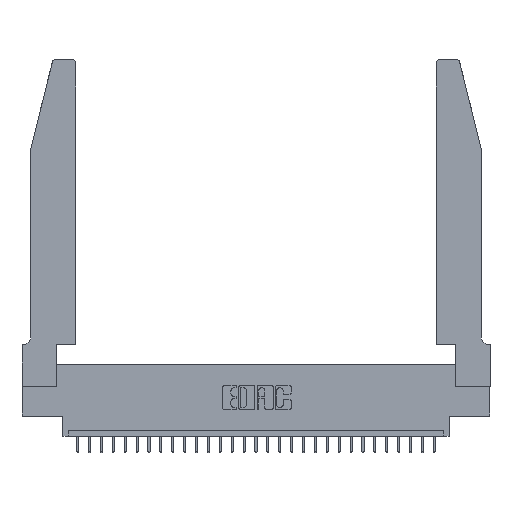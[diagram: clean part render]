
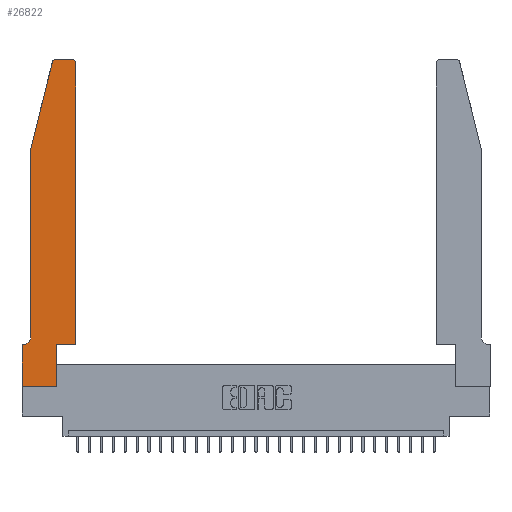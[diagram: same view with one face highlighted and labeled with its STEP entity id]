
A CAD part, top view. The second image highlights one B-rep face of the part: STEP entity #26822.
In plain terms, the highlighted planar face has unit normal (0, 0, 1).
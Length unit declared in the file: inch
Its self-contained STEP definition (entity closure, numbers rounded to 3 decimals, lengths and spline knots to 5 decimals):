
#91 = CARTESIAN_POINT ( 'NONE',  ( 0.4505, 0.35, 0.37 ) ) ;
#554 = CARTESIAN_POINT ( 'NONE',  ( 0.2865, 0.35, 0.37 ) ) ;
#603 = CARTESIAN_POINT ( 'NONE',  ( 0., 0., 0.37 ) ) ;
#962 = VECTOR ( 'NONE', #23819, 39.37008 ) ;
#1240 = VECTOR ( 'NONE', #25813, 39.37008 ) ;
#1410 = VECTOR ( 'NONE', #29481, 39.37008 ) ;
#1724 = ORIENTED_EDGE ( 'NONE', *, *, #6148, .T. ) ;
#1778 = DIRECTION ( 'NONE',  ( 0., 0., -1. ) ) ;
#2444 = PLANE ( 'NONE',  #16899 ) ;
#2586 = FACE_OUTER_BOUND ( 'NONE', #18977, .T. ) ;
#2711 = CARTESIAN_POINT ( 'NONE',  ( 0.284, 2.75, 0.37 ) ) ;
#2952 = DIRECTION ( 'NONE',  ( 1., 0., 0. ) ) ;
#3609 = CARTESIAN_POINT ( 'NONE',  ( 0.0055, 0.42, 0.37 ) ) ;
#3892 = DIRECTION ( 'NONE',  ( -1., 0., 0. ) ) ;
#3973 = VERTEX_POINT ( 'NONE', #24589 ) ;
#4111 = VERTEX_POINT ( 'NONE', #554 ) ;
#4314 = LINE ( 'NONE', #23002, #27967 ) ;
#4425 = CARTESIAN_POINT ( 'NONE',  ( 0.25487, 2.72718, 0.37 ) ) ;
#4513 = EDGE_CURVE ( 'NONE', #6541, #19945, #12818, .T. ) ;
#4769 = ORIENTED_EDGE ( 'NONE', *, *, #24061, .T. ) ;
#4992 = DIRECTION ( 'NONE',  ( 0., 0., 1. ) ) ;
#5116 = CARTESIAN_POINT ( 'NONE',  ( 0.2865, 0.35, 0.37 ) ) ;
#5364 = EDGE_CURVE ( 'NONE', #3973, #4111, #9200, .T. ) ;
#6148 = EDGE_CURVE ( 'NONE', #21252, #3973, #9681, .T. ) ;
#6361 = CARTESIAN_POINT ( 'NONE',  ( 0.284, 2.72, 0.37 ) ) ;
#6541 = VERTEX_POINT ( 'NONE', #2711 ) ;
#7515 = CARTESIAN_POINT ( 'NONE',  ( 0., 0.35, 0.37 ) ) ;
#7552 = LINE ( 'NONE', #603, #962 ) ;
#7604 = ORIENTED_EDGE ( 'NONE', *, *, #14848, .T. ) ;
#8193 = VECTOR ( 'NONE', #8995, 39.37008 ) ;
#8543 = VERTEX_POINT ( 'NONE', #29185 ) ;
#8554 = LINE ( 'NONE', #24541, #28881 ) ;
#8576 = CIRCLE ( 'NONE', #17254, 0.07 ) ;
#8995 = DIRECTION ( 'NONE',  ( 0., -1., 0. ) ) ;
#9142 = CARTESIAN_POINT ( 'NONE',  ( 0.0755, 2., 0.37 ) ) ;
#9200 = LINE ( 'NONE', #5116, #25303 ) ;
#9377 = CARTESIAN_POINT ( 'NONE',  ( 0., 0., 0.37 ) ) ;
#9437 = CARTESIAN_POINT ( 'NONE',  ( 0.0755, 2., 0.37 ) ) ;
#9579 = DIRECTION ( 'NONE',  ( 0., 0., 1. ) ) ;
#9681 = LINE ( 'NONE', #9377, #1240 ) ;
#9996 = VERTEX_POINT ( 'NONE', #29650 ) ;
#10591 = DIRECTION ( 'NONE',  ( 0., 0., 1. ) ) ;
#11072 = VERTEX_POINT ( 'NONE', #13559 ) ;
#11212 = VERTEX_POINT ( 'NONE', #7515 ) ;
#11536 = EDGE_CURVE ( 'NONE', #8543, #11212, #4314, .T. ) ;
#11781 = CARTESIAN_POINT ( 'NONE',  ( 0., 0.35, 0.37 ) ) ;
#12109 = EDGE_CURVE ( 'NONE', #11212, #21252, #7552, .T. ) ;
#12818 = CIRCLE ( 'NONE', #26299, 0.03 ) ;
#13132 = CARTESIAN_POINT ( 'NONE',  ( 0.0755, 0.42, 0.37 ) ) ;
#13311 = ORIENTED_EDGE ( 'NONE', *, *, #12109, .T. ) ;
#13559 = CARTESIAN_POINT ( 'NONE',  ( 0.4505, 2.72, 0.37 ) ) ;
#13827 = ORIENTED_EDGE ( 'NONE', *, *, #26193, .T. ) ;
#14027 = DIRECTION ( 'NONE',  ( 1., 0., 0. ) ) ;
#14195 = DIRECTION ( 'NONE',  ( 1., 0., 0. ) ) ;
#14410 = CARTESIAN_POINT ( 'NONE',  ( 0.4205, 2.72, 0.37 ) ) ;
#14848 = EDGE_CURVE ( 'NONE', #4111, #17467, #18849, .T. ) ;
#15706 = ORIENTED_EDGE ( 'NONE', *, *, #5364, .T. ) ;
#16241 = LINE ( 'NONE', #9437, #8193 ) ;
#16899 = AXIS2_PLACEMENT_3D ( 'NONE', #11781, #4992, #14195 ) ;
#16918 = ORIENTED_EDGE ( 'NONE', *, *, #11536, .T. ) ;
#17254 = AXIS2_PLACEMENT_3D ( 'NONE', #3609, #1778, #26675 ) ;
#17391 = DIRECTION ( 'NONE',  ( 1., 0., 0. ) ) ;
#17467 = VERTEX_POINT ( 'NONE', #17987 ) ;
#17499 = CARTESIAN_POINT ( 'NONE',  ( 0.0755, 2., 0.37 ) ) ;
#17935 = VECTOR ( 'NONE', #14027, 39.37008 ) ;
#17987 = CARTESIAN_POINT ( 'NONE',  ( 0.4505, 0.35, 0.37 ) ) ;
#18769 = AXIS2_PLACEMENT_3D ( 'NONE', #14410, #9579, #2952 ) ;
#18849 = LINE ( 'NONE', #23213, #17935 ) ;
#18977 = EDGE_LOOP ( 'NONE', ( #13827, #29520, #27305, #29112, #29342, #16918, #13311, #1724, #15706, #7604, #19452, #4769 ) ) ;
#19452 = ORIENTED_EDGE ( 'NONE', *, *, #23923, .T. ) ;
#19945 = VERTEX_POINT ( 'NONE', #4425 ) ;
#20305 = LINE ( 'NONE', #91, #1410 ) ;
#21252 = VERTEX_POINT ( 'NONE', #28728 ) ;
#22058 = EDGE_CURVE ( 'NONE', #25879, #8543, #8576, .T. ) ;
#23002 = CARTESIAN_POINT ( 'NONE',  ( 0.0755, 0.35, 0.37 ) ) ;
#23081 = CIRCLE ( 'NONE', #18769, 0.03 ) ;
#23099 = VECTOR ( 'NONE', #24717, 39.37008 ) ;
#23213 = CARTESIAN_POINT ( 'NONE',  ( 0.4505, 0.35, 0.37 ) ) ;
#23353 = DIRECTION ( 'NONE',  ( 0., 1., 0. ) ) ;
#23819 = DIRECTION ( 'NONE',  ( 0., -1., 0. ) ) ;
#23901 = VERTEX_POINT ( 'NONE', #9142 ) ;
#23923 = EDGE_CURVE ( 'NONE', #17467, #11072, #20305, .T. ) ;
#24061 = EDGE_CURVE ( 'NONE', #11072, #9996, #23081, .T. ) ;
#24420 = LINE ( 'NONE', #17499, #23099 ) ;
#24541 = CARTESIAN_POINT ( 'NONE',  ( 0.2605, 2.75, 0.37 ) ) ;
#24589 = CARTESIAN_POINT ( 'NONE',  ( 0.2865, 0., 0.37 ) ) ;
#24717 = DIRECTION ( 'NONE',  ( -0.239, -0.971, 0. ) ) ;
#25303 = VECTOR ( 'NONE', #23353, 39.37008 ) ;
#25796 = EDGE_CURVE ( 'NONE', #19945, #23901, #24420, .T. ) ;
#25813 = DIRECTION ( 'NONE',  ( 1., 0., 0. ) ) ;
#25879 = VERTEX_POINT ( 'NONE', #13132 ) ;
#26193 = EDGE_CURVE ( 'NONE', #9996, #6541, #8554, .T. ) ;
#26299 = AXIS2_PLACEMENT_3D ( 'NONE', #6361, #10591, #17391 ) ;
#26343 = EDGE_CURVE ( 'NONE', #23901, #25879, #16241, .T. ) ;
#26675 = DIRECTION ( 'NONE',  ( -1., 0., 0. ) ) ;
#26822 = ADVANCED_FACE ( 'NONE', ( #2586 ), #2444, .T. ) ;
#27305 = ORIENTED_EDGE ( 'NONE', *, *, #25796, .T. ) ;
#27371 = DIRECTION ( 'NONE',  ( -1., 0., 0. ) ) ;
#27967 = VECTOR ( 'NONE', #27371, 39.37008 ) ;
#28728 = CARTESIAN_POINT ( 'NONE',  ( 0., 0., 0.37 ) ) ;
#28881 = VECTOR ( 'NONE', #3892, 39.37008 ) ;
#29112 = ORIENTED_EDGE ( 'NONE', *, *, #26343, .T. ) ;
#29185 = CARTESIAN_POINT ( 'NONE',  ( 0.0055, 0.35, 0.37 ) ) ;
#29342 = ORIENTED_EDGE ( 'NONE', *, *, #22058, .T. ) ;
#29481 = DIRECTION ( 'NONE',  ( 0., 1., 0. ) ) ;
#29520 = ORIENTED_EDGE ( 'NONE', *, *, #4513, .T. ) ;
#29650 = CARTESIAN_POINT ( 'NONE',  ( 0.4205, 2.75, 0.37 ) ) ;
